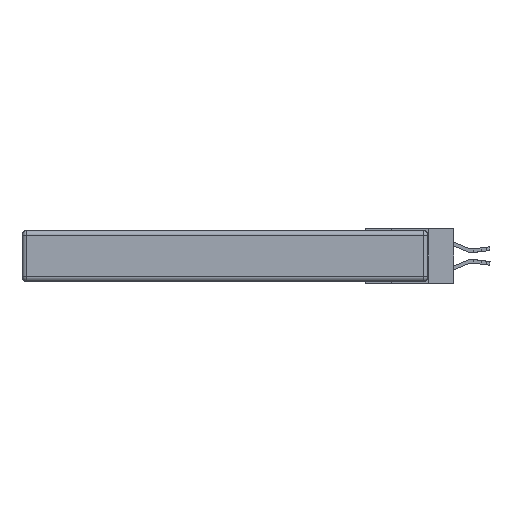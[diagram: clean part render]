
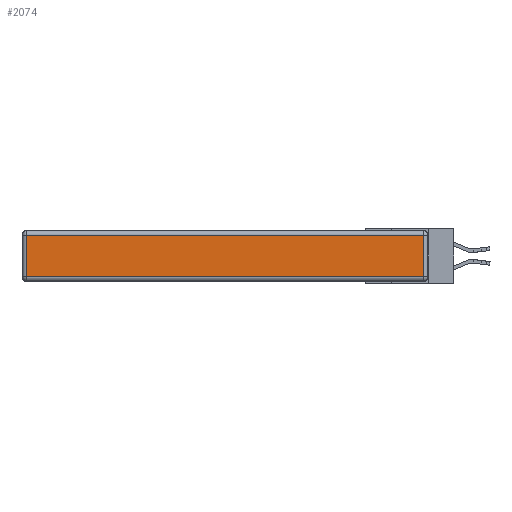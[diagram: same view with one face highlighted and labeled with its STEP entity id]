
A CAD part, left-side view. The second image highlights one B-rep face of the part: STEP entity #2074.
In plain terms, the highlighted planar face has unit normal (-1, 0, 0).
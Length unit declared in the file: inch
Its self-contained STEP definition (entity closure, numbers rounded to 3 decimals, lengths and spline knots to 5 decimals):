
#780 = ORIENTED_EDGE ( 'NONE', *, *, #3733, .T. ) ;
#1988 = VECTOR ( 'NONE', #9859, 39.37008 ) ;
#2062 = VERTEX_POINT ( 'NONE', #19215 ) ;
#2074 = ADVANCED_FACE ( 'NONE', ( #22217 ), #14147, .T. ) ;
#2563 = EDGE_CURVE ( 'NONE', #15710, #3788, #21916, .T. ) ;
#3733 = EDGE_CURVE ( 'NONE', #3788, #2062, #7664, .T. ) ;
#3788 = VERTEX_POINT ( 'NONE', #16910 ) ;
#4984 = AXIS2_PLACEMENT_3D ( 'NONE', #5141, #21346, #23022 ) ;
#5141 = CARTESIAN_POINT ( 'NONE',  ( 0., 0., -0.343 ) ) ;
#5945 = CARTESIAN_POINT ( 'NONE',  ( 0., 0.03, -0.343 ) ) ;
#6547 = VECTOR ( 'NONE', #18567, 39.37008 ) ;
#7373 = CARTESIAN_POINT ( 'NONE',  ( 0., 2.75, -0.03 ) ) ;
#7664 = LINE ( 'NONE', #7373, #18486 ) ;
#7787 = DIRECTION ( 'NONE',  ( 0., 0., 1. ) ) ;
#7823 = VERTEX_POINT ( 'NONE', #10541 ) ;
#7964 = LINE ( 'NONE', #18410, #6547 ) ;
#8590 = VECTOR ( 'NONE', #7787, 39.37008 ) ;
#9396 = LINE ( 'NONE', #15547, #1988 ) ;
#9859 = DIRECTION ( 'NONE',  ( 0., 0., -1. ) ) ;
#10541 = CARTESIAN_POINT ( 'NONE',  ( 0., 2.72, -0.313 ) ) ;
#13996 = ORIENTED_EDGE ( 'NONE', *, *, #14818, .T. ) ;
#14147 = PLANE ( 'NONE',  #4984 ) ;
#14818 = EDGE_CURVE ( 'NONE', #7823, #15710, #7964, .T. ) ;
#15480 = ORIENTED_EDGE ( 'NONE', *, *, #2563, .T. ) ;
#15547 = CARTESIAN_POINT ( 'NONE',  ( 0., 2.72, -0.343 ) ) ;
#15710 = VERTEX_POINT ( 'NONE', #19516 ) ;
#16745 = DIRECTION ( 'NONE',  ( 0., 1., 0. ) ) ;
#16910 = CARTESIAN_POINT ( 'NONE',  ( 0., 0.03, -0.03 ) ) ;
#17260 = EDGE_LOOP ( 'NONE', ( #13996, #15480, #780, #23034 ) ) ;
#18410 = CARTESIAN_POINT ( 'NONE',  ( 0., 0., -0.313 ) ) ;
#18486 = VECTOR ( 'NONE', #16745, 39.37008 ) ;
#18567 = DIRECTION ( 'NONE',  ( 0., -1., 0. ) ) ;
#19215 = CARTESIAN_POINT ( 'NONE',  ( 0., 2.72, -0.03 ) ) ;
#19516 = CARTESIAN_POINT ( 'NONE',  ( 0., 0.03, -0.313 ) ) ;
#21346 = DIRECTION ( 'NONE',  ( -1., 0., 0. ) ) ;
#21916 = LINE ( 'NONE', #5945, #8590 ) ;
#22184 = EDGE_CURVE ( 'NONE', #2062, #7823, #9396, .T. ) ;
#22217 = FACE_OUTER_BOUND ( 'NONE', #17260, .T. ) ;
#23022 = DIRECTION ( 'NONE',  ( 0., 0., 1. ) ) ;
#23034 = ORIENTED_EDGE ( 'NONE', *, *, #22184, .T. ) ;
